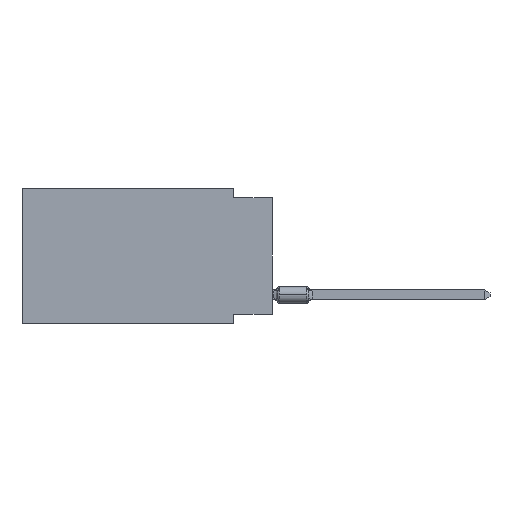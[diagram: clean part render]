
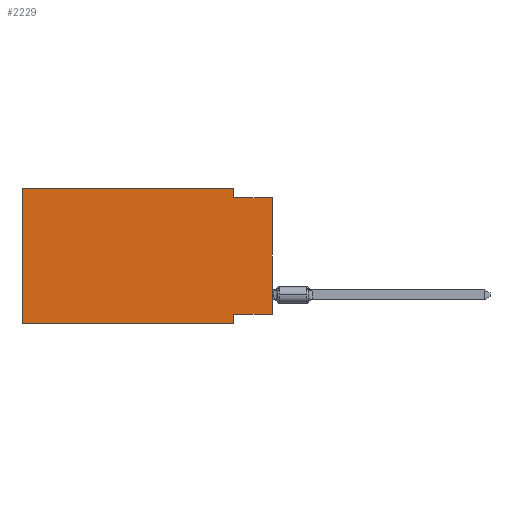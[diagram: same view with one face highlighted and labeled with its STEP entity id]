
A CAD part, left-side view. The second image highlights one B-rep face of the part: STEP entity #2229.
In plain terms, the highlighted planar face has unit normal (-1, 0, 0).
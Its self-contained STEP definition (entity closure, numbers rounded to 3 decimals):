
#330 = VERTEX_POINT ( 'NONE', #6918 ) ;
#425 = VERTEX_POINT ( 'NONE', #4104 ) ;
#593 = LINE ( 'NONE', #8810, #10648 ) ;
#1442 = VERTEX_POINT ( 'NONE', #4484 ) ;
#1521 = EDGE_CURVE ( 'NONE', #330, #1442, #9194, .T. ) ;
#1740 = EDGE_CURVE ( 'NONE', #12904, #4504, #12075, .T. ) ;
#1913 = ORIENTED_EDGE ( 'NONE', *, *, #1740, .F. ) ;
#1960 = VERTEX_POINT ( 'NONE', #6823 ) ;
#2037 = DIRECTION ( 'NONE',  ( 0., 0., 1. ) ) ;
#2123 = VECTOR ( 'NONE', #12441, 1000. ) ;
#2229 = ADVANCED_FACE ( 'NONE', ( #8723 ), #13348, .F. ) ;
#2276 = DIRECTION ( 'NONE',  ( 0., -1., 0. ) ) ;
#2871 = ORIENTED_EDGE ( 'NONE', *, *, #7699, .F. ) ;
#2948 = CARTESIAN_POINT ( 'NONE',  ( 0., 16.383, 0. ) ) ;
#3213 = EDGE_CURVE ( 'NONE', #330, #7443, #13874, .T. ) ;
#3382 = LINE ( 'NONE', #10170, #2123 ) ;
#3807 = ORIENTED_EDGE ( 'NONE', *, *, #1521, .T. ) ;
#3945 = CARTESIAN_POINT ( 'NONE',  ( 0., 0., -0.635 ) ) ;
#4104 = CARTESIAN_POINT ( 'NONE',  ( 0., 2.54, 0. ) ) ;
#4236 = DIRECTION ( 'NONE',  ( 0., 1., 0. ) ) ;
#4484 = CARTESIAN_POINT ( 'NONE',  ( 0., 2.54, -8.89 ) ) ;
#4504 = VERTEX_POINT ( 'NONE', #13896 ) ;
#4935 = CARTESIAN_POINT ( 'NONE',  ( 0., 0., 0. ) ) ;
#5423 = VECTOR ( 'NONE', #8417, 1000. ) ;
#5501 = EDGE_LOOP ( 'NONE', ( #9356, #1913, #14611, #13582, #13045, #3807, #6435, #2871 ) ) ;
#5610 = VECTOR ( 'NONE', #7596, 1000. ) ;
#5866 = DIRECTION ( 'NONE',  ( 0., 0., -1. ) ) ;
#6435 = ORIENTED_EDGE ( 'NONE', *, *, #6610, .F. ) ;
#6442 = DIRECTION ( 'NONE',  ( 1., 0., 0. ) ) ;
#6567 = VERTEX_POINT ( 'NONE', #12583 ) ;
#6610 = EDGE_CURVE ( 'NONE', #1960, #1442, #3382, .T. ) ;
#6765 = VECTOR ( 'NONE', #2037, 1000. ) ;
#6823 = CARTESIAN_POINT ( 'NONE',  ( 0., 2.54, -8.255 ) ) ;
#6918 = CARTESIAN_POINT ( 'NONE',  ( 0., 16.383, -8.89 ) ) ;
#7443 = VERTEX_POINT ( 'NONE', #12971 ) ;
#7596 = DIRECTION ( 'NONE',  ( 0., -1., 0. ) ) ;
#7699 = EDGE_CURVE ( 'NONE', #6567, #1960, #12292, .T. ) ;
#8108 = LINE ( 'NONE', #4935, #5423 ) ;
#8136 = CARTESIAN_POINT ( 'NONE',  ( 0., 2.54, 0. ) ) ;
#8417 = DIRECTION ( 'NONE',  ( 0., 0., 1. ) ) ;
#8538 = VECTOR ( 'NONE', #5866, 1000. ) ;
#8723 = FACE_OUTER_BOUND ( 'NONE', #5501, .T. ) ;
#8810 = CARTESIAN_POINT ( 'NONE',  ( 0., 16.383, 0. ) ) ;
#9141 = EDGE_CURVE ( 'NONE', #425, #12904, #12626, .T. ) ;
#9194 = LINE ( 'NONE', #11632, #10211 ) ;
#9356 = ORIENTED_EDGE ( 'NONE', *, *, #13872, .T. ) ;
#9829 = EDGE_CURVE ( 'NONE', #7443, #425, #593, .T. ) ;
#10031 = CARTESIAN_POINT ( 'NONE',  ( 0., 0., -8.255 ) ) ;
#10170 = CARTESIAN_POINT ( 'NONE',  ( 0., 2.54, -8.89 ) ) ;
#10211 = VECTOR ( 'NONE', #2276, 1000. ) ;
#10648 = VECTOR ( 'NONE', #12294, 1000. ) ;
#11632 = CARTESIAN_POINT ( 'NONE',  ( 0., 16.383, -8.89 ) ) ;
#12075 = LINE ( 'NONE', #3945, #5610 ) ;
#12292 = LINE ( 'NONE', #10031, #14991 ) ;
#12294 = DIRECTION ( 'NONE',  ( 0., -1., 0. ) ) ;
#12441 = DIRECTION ( 'NONE',  ( 0., 0., -1. ) ) ;
#12521 = CARTESIAN_POINT ( 'NONE',  ( 0., 16.383, 0. ) ) ;
#12583 = CARTESIAN_POINT ( 'NONE',  ( 0., 0., -8.255 ) ) ;
#12626 = LINE ( 'NONE', #8136, #8538 ) ;
#12904 = VERTEX_POINT ( 'NONE', #13326 ) ;
#12971 = CARTESIAN_POINT ( 'NONE',  ( 0., 16.383, 0. ) ) ;
#13045 = ORIENTED_EDGE ( 'NONE', *, *, #3213, .F. ) ;
#13101 = AXIS2_PLACEMENT_3D ( 'NONE', #2948, #6442, #14684 ) ;
#13326 = CARTESIAN_POINT ( 'NONE',  ( 0., 2.54, -0.635 ) ) ;
#13348 = PLANE ( 'NONE',  #13101 ) ;
#13582 = ORIENTED_EDGE ( 'NONE', *, *, #9829, .F. ) ;
#13872 = EDGE_CURVE ( 'NONE', #6567, #4504, #8108, .T. ) ;
#13874 = LINE ( 'NONE', #12521, #6765 ) ;
#13896 = CARTESIAN_POINT ( 'NONE',  ( 0., 0., -0.635 ) ) ;
#14611 = ORIENTED_EDGE ( 'NONE', *, *, #9141, .F. ) ;
#14684 = DIRECTION ( 'NONE',  ( 0., 0., -1. ) ) ;
#14991 = VECTOR ( 'NONE', #4236, 1000. ) ;
